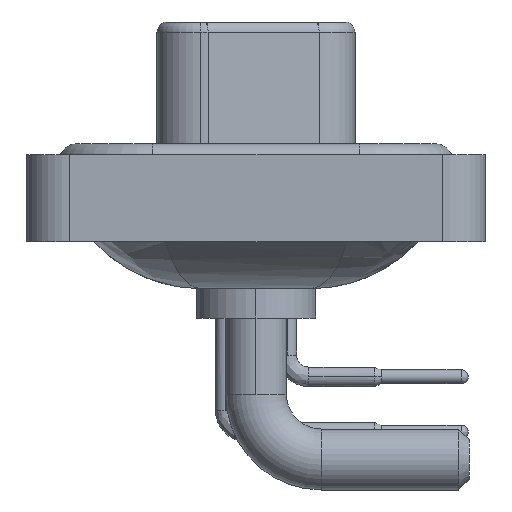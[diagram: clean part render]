
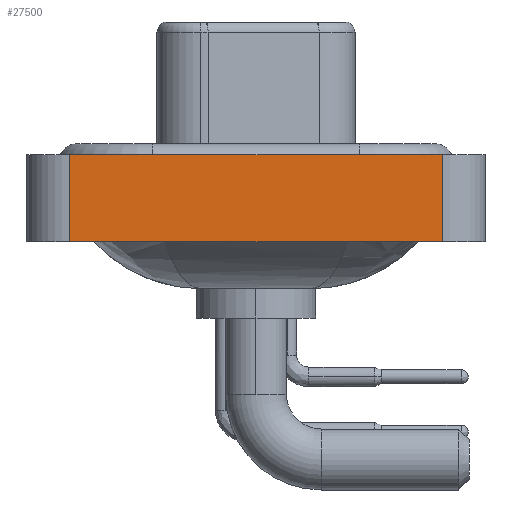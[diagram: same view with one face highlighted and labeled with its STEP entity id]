
A CAD part, left-side view. The second image highlights one B-rep face of the part: STEP entity #27500.
In plain terms, the highlighted planar face has unit normal (-1, 0, 0).
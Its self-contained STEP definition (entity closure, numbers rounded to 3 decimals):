
#2181 = CARTESIAN_POINT ( 'NONE',  ( -7.35, 8.55, -3.6 ) ) ;
#2554 = VECTOR ( 'NONE', #21956, 1000. ) ;
#2950 = DIRECTION ( 'NONE',  ( 0., 0., 1. ) ) ;
#4038 = EDGE_CURVE ( 'NONE', #14415, #20896, #17741, .T. ) ;
#4097 = CARTESIAN_POINT ( 'NONE',  ( -7.35, -8.55, -3.6 ) ) ;
#4510 = VECTOR ( 'NONE', #17614, 1000. ) ;
#4753 = ORIENTED_EDGE ( 'NONE', *, *, #6922, .T. ) ;
#5253 = EDGE_CURVE ( 'NONE', #25838, #5995, #23851, .T. ) ;
#5376 = CARTESIAN_POINT ( 'NONE',  ( -7.35, -8.55, -3.6 ) ) ;
#5995 = VERTEX_POINT ( 'NONE', #16411 ) ;
#6922 = EDGE_CURVE ( 'NONE', #14415, #25838, #27395, .T. ) ;
#8291 = CARTESIAN_POINT ( 'NONE',  ( -7.35, 8.55, -3.6 ) ) ;
#9613 = EDGE_LOOP ( 'NONE', ( #10201, #26260, #23715, #4753 ) ) ;
#10201 = ORIENTED_EDGE ( 'NONE', *, *, #5253, .T. ) ;
#13559 = EDGE_CURVE ( 'NONE', #20896, #5995, #27651, .T. ) ;
#13983 = CARTESIAN_POINT ( 'NONE',  ( -7.35, -8.55, -3.6 ) ) ;
#14415 = VERTEX_POINT ( 'NONE', #8291 ) ;
#14545 = AXIS2_PLACEMENT_3D ( 'NONE', #5376, #20545, #2950 ) ;
#16411 = CARTESIAN_POINT ( 'NONE',  ( -7.35, -8.55, 0.4 ) ) ;
#17614 = DIRECTION ( 'NONE',  ( 0., 0., 1. ) ) ;
#17741 = LINE ( 'NONE', #2181, #4510 ) ;
#18039 = VECTOR ( 'NONE', #25257, 1000. ) ;
#18520 = PLANE ( 'NONE',  #14545 ) ;
#18710 = DIRECTION ( 'NONE',  ( 0., -1., 0. ) ) ;
#20254 = VECTOR ( 'NONE', #18710, 1000. ) ;
#20545 = DIRECTION ( 'NONE',  ( -1., 0., 0. ) ) ;
#20896 = VERTEX_POINT ( 'NONE', #21960 ) ;
#21956 = DIRECTION ( 'NONE',  ( 0., 0., 1. ) ) ;
#21960 = CARTESIAN_POINT ( 'NONE',  ( -7.35, 8.55, 0.4 ) ) ;
#22699 = FACE_OUTER_BOUND ( 'NONE', #9613, .T. ) ;
#23350 = CARTESIAN_POINT ( 'NONE',  ( -7.35, -8.55, 0.4 ) ) ;
#23715 = ORIENTED_EDGE ( 'NONE', *, *, #4038, .F. ) ;
#23851 = LINE ( 'NONE', #4097, #2554 ) ;
#25257 = DIRECTION ( 'NONE',  ( 0., -1., 0. ) ) ;
#25838 = VERTEX_POINT ( 'NONE', #27750 ) ;
#26260 = ORIENTED_EDGE ( 'NONE', *, *, #13559, .F. ) ;
#27395 = LINE ( 'NONE', #13983, #18039 ) ;
#27500 = ADVANCED_FACE ( 'NONE', ( #22699 ), #18520, .T. ) ;
#27651 = LINE ( 'NONE', #23350, #20254 ) ;
#27750 = CARTESIAN_POINT ( 'NONE',  ( -7.35, -8.55, -3.6 ) ) ;
